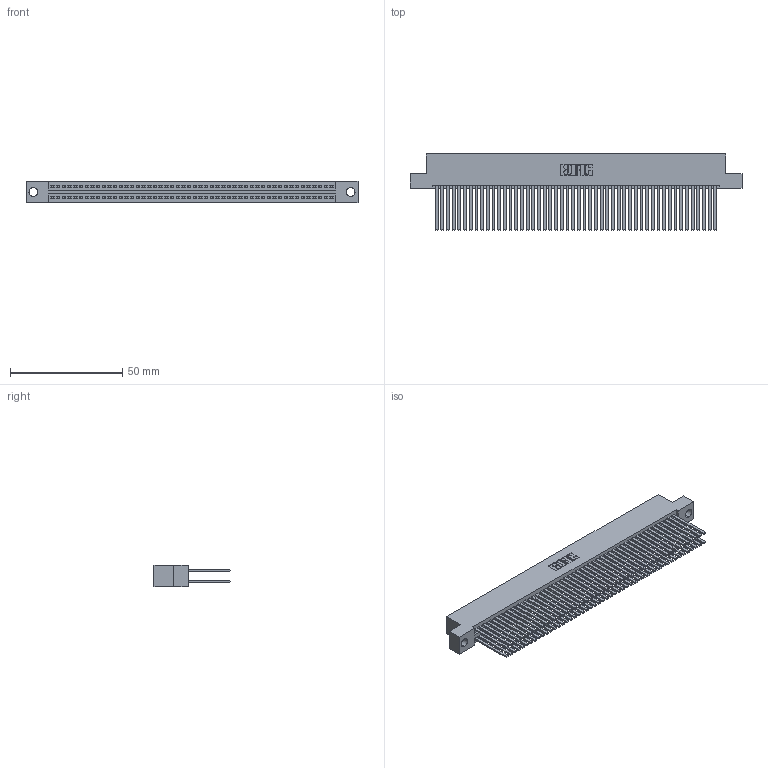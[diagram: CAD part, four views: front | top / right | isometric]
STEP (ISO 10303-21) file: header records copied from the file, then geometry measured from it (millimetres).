
FILE_DESCRIPTION (( 'STEP AP203' ), '1' );
FILE_NAME ('345-100-544-204.STEP', '2018-10-05T15:46:55', ( '' ), ( '' ), 'SwSTEP 2.0', 'SolidWorks 2016', '' );
FILE_SCHEMA (( 'CONFIG_CONTROL_DESIGN' ));
Length unit declared in the file: inch
Products named in the file (3): 345-292-001_345-293-144; 345-100-544-204; 345 Part_Flush Mounting Lugs - 0.156 Dia-TH
Assembly tree (101 placements, depth 2):
  345-100-544-204
    345 Part_Flush Mounting Lugs - 0.156 Dia-TH
    345-292-001_345-293-144  x100
Bounding box: 148.21 x 33.96 x 9.4 mm (x, y, z)
Volume: 15785.4 mm3; surface area: 27412.2 mm2
Topology: 101 solids, 101 shells, 4526 faces, 13441 edges, 8826 vertices
Faces by surface type: plane 2980, cylinder 1546
Entity records: 37973 total; most frequent: CARTESIAN_POINT 6356, ORIENTED_EDGE 6290, DIRECTION 5593, EDGE_CURVE 3145, VECTOR 2817, LINE 2817, VERTEX_POINT 2094, AXIS2_PLACEMENT_3D 1388
